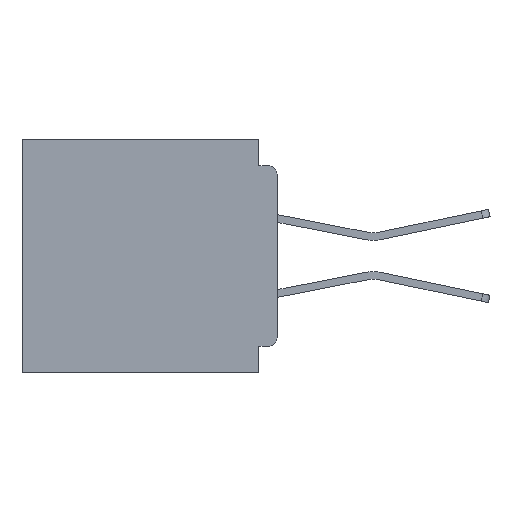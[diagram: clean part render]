
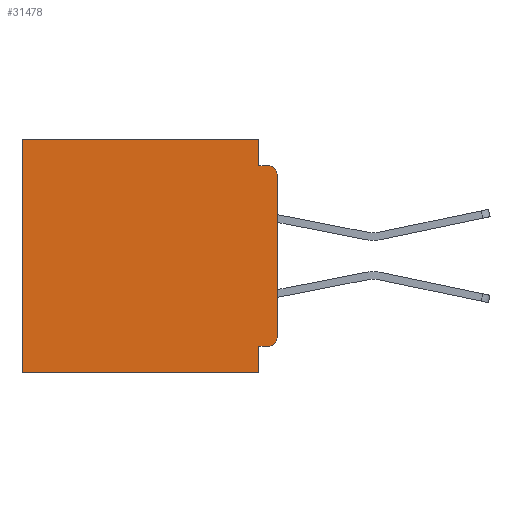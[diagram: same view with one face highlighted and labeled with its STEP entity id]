
A CAD part, left-side view. The second image highlights one B-rep face of the part: STEP entity #31478.
In plain terms, the highlighted planar face has unit normal (-1, 0, 0).
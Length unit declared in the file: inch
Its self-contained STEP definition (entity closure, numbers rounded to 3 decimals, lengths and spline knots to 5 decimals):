
#733 = LINE ( 'NONE', #42125, #23741 ) ;
#2509 = CARTESIAN_POINT ( 'NONE',  ( 0.3, 0., -0.355 ) ) ;
#3614 = DIRECTION ( 'NONE',  ( 1., 0., 0. ) ) ;
#3756 = VECTOR ( 'NONE', #15323, 39.37008 ) ;
#3906 = ORIENTED_EDGE ( 'NONE', *, *, #12309, .T. ) ;
#4107 = CARTESIAN_POINT ( 'NONE',  ( 0.3, 0.437, 0. ) ) ;
#4256 = CARTESIAN_POINT ( 'NONE',  ( 0.3, 0., -0.06 ) ) ;
#5156 = FACE_OUTER_BOUND ( 'NONE', #10050, .T. ) ;
#6643 = CARTESIAN_POINT ( 'NONE',  ( 0.3, 0., -0.045 ) ) ;
#7360 = CARTESIAN_POINT ( 'NONE',  ( 0.3, 0.437, -0.4 ) ) ;
#7874 = DIRECTION ( 'NONE',  ( -1., 0., 0. ) ) ;
#7938 = CARTESIAN_POINT ( 'NONE',  ( 0.3, 0.015, -0.355 ) ) ;
#8479 = ORIENTED_EDGE ( 'NONE', *, *, #29526, .F. ) ;
#9702 = CARTESIAN_POINT ( 'NONE',  ( 0.3, 0.031, -0.355 ) ) ;
#9851 = DIRECTION ( 'NONE',  ( -1., 0., 0. ) ) ;
#10015 = LINE ( 'NONE', #35453, #20776 ) ;
#10050 = EDGE_LOOP ( 'NONE', ( #19291, #3906, #26535, #8479, #54398, #34982, #39457, #43368, #31027, #39389 ) ) ;
#10457 = VECTOR ( 'NONE', #51739, 39.37008 ) ;
#10514 = CARTESIAN_POINT ( 'NONE',  ( 0.3, 0., -0.4 ) ) ;
#12309 = EDGE_CURVE ( 'NONE', #42124, #55664, #27971, .T. ) ;
#12577 = DIRECTION ( 'NONE',  ( 0., 0., -1. ) ) ;
#13495 = VERTEX_POINT ( 'NONE', #7938 ) ;
#13594 = VECTOR ( 'NONE', #46183, 39.37008 ) ;
#15323 = DIRECTION ( 'NONE',  ( 0., 1., 0. ) ) ;
#15960 = LINE ( 'NONE', #47383, #3756 ) ;
#16063 = EDGE_CURVE ( 'NONE', #42124, #33716, #733, .T. ) ;
#16852 = EDGE_CURVE ( 'NONE', #49025, #55664, #40967, .T. ) ;
#17434 = CARTESIAN_POINT ( 'NONE',  ( 0.3, 0.031, -0.4 ) ) ;
#19291 = ORIENTED_EDGE ( 'NONE', *, *, #16063, .F. ) ;
#19480 = CARTESIAN_POINT ( 'NONE',  ( 0.3, 0., -0.34 ) ) ;
#20216 = EDGE_CURVE ( 'NONE', #23661, #37560, #38046, .T. ) ;
#20776 = VECTOR ( 'NONE', #12577, 39.37008 ) ;
#20990 = DIRECTION ( 'NONE',  ( 0., 1., 0. ) ) ;
#21642 = EDGE_CURVE ( 'NONE', #13495, #27670, #53519, .T. ) ;
#21922 = PLANE ( 'NONE',  #26803 ) ;
#22687 = LINE ( 'NONE', #10514, #10457 ) ;
#23362 = CARTESIAN_POINT ( 'NONE',  ( 0.3, 0.031, 0. ) ) ;
#23661 = VERTEX_POINT ( 'NONE', #4107 ) ;
#23741 = VECTOR ( 'NONE', #28470, 39.37008 ) ;
#25817 = VECTOR ( 'NONE', #59209, 39.37008 ) ;
#26535 = ORIENTED_EDGE ( 'NONE', *, *, #16852, .F. ) ;
#26803 = AXIS2_PLACEMENT_3D ( 'NONE', #31178, #3614, #35762 ) ;
#26821 = EDGE_CURVE ( 'NONE', #33977, #23661, #15960, .T. ) ;
#27670 = VERTEX_POINT ( 'NONE', #9702 ) ;
#27971 = CIRCLE ( 'NONE', #55770, 0.015 ) ;
#28470 = DIRECTION ( 'NONE',  ( 0., 0., -1. ) ) ;
#29526 = EDGE_CURVE ( 'NONE', #33977, #49025, #50104, .T. ) ;
#31027 = ORIENTED_EDGE ( 'NONE', *, *, #21642, .F. ) ;
#31178 = CARTESIAN_POINT ( 'NONE',  ( 0.3, 0., -0.4 ) ) ;
#31478 = ADVANCED_FACE ( 'NONE', ( #5156 ), #21922, .F. ) ;
#32626 = EDGE_CURVE ( 'NONE', #27670, #53020, #10015, .T. ) ;
#33716 = VERTEX_POINT ( 'NONE', #19480 ) ;
#33977 = VERTEX_POINT ( 'NONE', #45133 ) ;
#34194 = DIRECTION ( 'NONE',  ( 0., -1., 0. ) ) ;
#34982 = ORIENTED_EDGE ( 'NONE', *, *, #20216, .T. ) ;
#35397 = CARTESIAN_POINT ( 'NONE',  ( 0.3, 0.015, -0.34 ) ) ;
#35453 = CARTESIAN_POINT ( 'NONE',  ( 0.3, 0.031, -0.4 ) ) ;
#35762 = DIRECTION ( 'NONE',  ( 0., 0., -1. ) ) ;
#36545 = CARTESIAN_POINT ( 'NONE',  ( 0.3, 0.437, -0.4 ) ) ;
#37334 = CARTESIAN_POINT ( 'NONE',  ( 0.3, 0.015, -0.06 ) ) ;
#37560 = VERTEX_POINT ( 'NONE', #7360 ) ;
#37849 = CIRCLE ( 'NONE', #42153, 0.015 ) ;
#38046 = LINE ( 'NONE', #36545, #25817 ) ;
#39389 = ORIENTED_EDGE ( 'NONE', *, *, #43948, .T. ) ;
#39457 = ORIENTED_EDGE ( 'NONE', *, *, #52084, .F. ) ;
#39524 = VECTOR ( 'NONE', #34194, 39.37008 ) ;
#40024 = DIRECTION ( 'NONE',  ( 0., 0., -1. ) ) ;
#40967 = LINE ( 'NONE', #6643, #39524 ) ;
#41463 = VECTOR ( 'NONE', #20990, 39.37008 ) ;
#41976 = DIRECTION ( 'NONE',  ( 0., 0., -1. ) ) ;
#42124 = VERTEX_POINT ( 'NONE', #4256 ) ;
#42125 = CARTESIAN_POINT ( 'NONE',  ( 0.3, 0., -0.4 ) ) ;
#42153 = AXIS2_PLACEMENT_3D ( 'NONE', #35397, #7874, #40024 ) ;
#43368 = ORIENTED_EDGE ( 'NONE', *, *, #32626, .F. ) ;
#43948 = EDGE_CURVE ( 'NONE', #13495, #33716, #37849, .T. ) ;
#45133 = CARTESIAN_POINT ( 'NONE',  ( 0.3, 0.031, 0. ) ) ;
#46183 = DIRECTION ( 'NONE',  ( 0., 0., -1. ) ) ;
#47383 = CARTESIAN_POINT ( 'NONE',  ( 0.3, 0., 0. ) ) ;
#49025 = VERTEX_POINT ( 'NONE', #51001 ) ;
#50104 = LINE ( 'NONE', #23362, #13594 ) ;
#51001 = CARTESIAN_POINT ( 'NONE',  ( 0.3, 0.031, -0.045 ) ) ;
#51739 = DIRECTION ( 'NONE',  ( 0., 1., 0. ) ) ;
#52084 = EDGE_CURVE ( 'NONE', #53020, #37560, #22687, .T. ) ;
#53020 = VERTEX_POINT ( 'NONE', #17434 ) ;
#53063 = CARTESIAN_POINT ( 'NONE',  ( 0.3, 0.015, -0.045 ) ) ;
#53519 = LINE ( 'NONE', #2509, #41463 ) ;
#54398 = ORIENTED_EDGE ( 'NONE', *, *, #26821, .T. ) ;
#55664 = VERTEX_POINT ( 'NONE', #53063 ) ;
#55770 = AXIS2_PLACEMENT_3D ( 'NONE', #37334, #9851, #41976 ) ;
#59209 = DIRECTION ( 'NONE',  ( 0., 0., -1. ) ) ;
